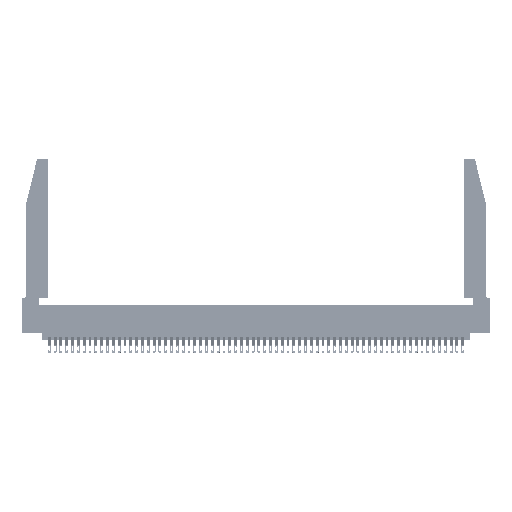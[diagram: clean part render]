
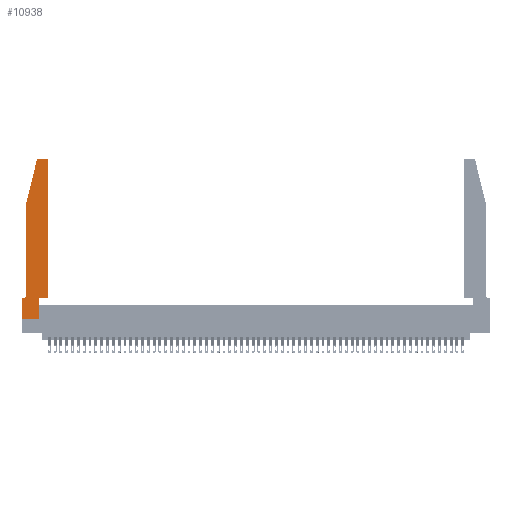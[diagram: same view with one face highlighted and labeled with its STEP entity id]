
A CAD part, top view. The second image highlights one B-rep face of the part: STEP entity #10938.
In plain terms, the highlighted planar face has unit normal (0, 0, 1).
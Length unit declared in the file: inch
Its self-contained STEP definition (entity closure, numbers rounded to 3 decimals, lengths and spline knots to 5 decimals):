
#44 = EDGE_CURVE ( 'NONE', #14950, #2141, #17906, .T. ) ;
#338 = EDGE_CURVE ( 'NONE', #9781, #14950, #34547, .T. ) ;
#500 = ORIENTED_EDGE ( 'NONE', *, *, #44272, .T. ) ;
#587 = DIRECTION ( 'NONE',  ( 1., 0., 0. ) ) ;
#1135 = CARTESIAN_POINT ( 'NONE',  ( 0.0055, 0.35, 0.37 ) ) ;
#1324 = ORIENTED_EDGE ( 'NONE', *, *, #37859, .T. ) ;
#2141 = VERTEX_POINT ( 'NONE', #27934 ) ;
#2411 = EDGE_CURVE ( 'NONE', #54295, #3320, #35051, .T. ) ;
#2538 = ORIENTED_EDGE ( 'NONE', *, *, #2411, .T. ) ;
#2945 = VERTEX_POINT ( 'NONE', #25527 ) ;
#3294 = DIRECTION ( 'NONE',  ( 0., 1., 0. ) ) ;
#3320 = VERTEX_POINT ( 'NONE', #22599 ) ;
#3808 = ORIENTED_EDGE ( 'NONE', *, *, #50352, .T. ) ;
#4042 = CIRCLE ( 'NONE', #40705, 0.03 ) ;
#4461 = VECTOR ( 'NONE', #3294, 39.37008 ) ;
#5425 = CARTESIAN_POINT ( 'NONE',  ( 0., 0.35, 0.37 ) ) ;
#9781 = VERTEX_POINT ( 'NONE', #45982 ) ;
#9807 = EDGE_CURVE ( 'NONE', #54959, #39110, #18823, .T. ) ;
#10004 = CIRCLE ( 'NONE', #13353, 0.07 ) ;
#10031 = CARTESIAN_POINT ( 'NONE',  ( 0.0755, 2., 0.37 ) ) ;
#10104 = CARTESIAN_POINT ( 'NONE',  ( 0.4505, 0.35, 0.37 ) ) ;
#10716 = CARTESIAN_POINT ( 'NONE',  ( 0.25487, 2.72718, 0.37 ) ) ;
#10938 = ADVANCED_FACE ( 'NONE', ( #11097 ), #18618, .T. ) ;
#11097 = FACE_OUTER_BOUND ( 'NONE', #32152, .T. ) ;
#13084 = LINE ( 'NONE', #56034, #25462 ) ;
#13353 = AXIS2_PLACEMENT_3D ( 'NONE', #24108, #41771, #50755 ) ;
#13723 = DIRECTION ( 'NONE',  ( 0., -1., 0. ) ) ;
#14192 = CARTESIAN_POINT ( 'NONE',  ( 0.4505, 0.35, 0.37 ) ) ;
#14578 = VECTOR ( 'NONE', #18341, 39.37008 ) ;
#14950 = VERTEX_POINT ( 'NONE', #10716 ) ;
#15101 = DIRECTION ( 'NONE',  ( 1., 0., 0. ) ) ;
#15201 = LINE ( 'NONE', #34002, #32562 ) ;
#17906 = LINE ( 'NONE', #43061, #54844 ) ;
#17944 = ORIENTED_EDGE ( 'NONE', *, *, #9807, .T. ) ;
#18142 = CARTESIAN_POINT ( 'NONE',  ( 0.284, 2.72, 0.37 ) ) ;
#18341 = DIRECTION ( 'NONE',  ( 0., 1., 0. ) ) ;
#18618 = PLANE ( 'NONE',  #49886 ) ;
#18672 = ORIENTED_EDGE ( 'NONE', *, *, #38114, .T. ) ;
#18814 = DIRECTION ( 'NONE',  ( 0., 0., 1. ) ) ;
#18823 = LINE ( 'NONE', #24023, #29229 ) ;
#18865 = DIRECTION ( 'NONE',  ( 1., 0., 0. ) ) ;
#19531 = DIRECTION ( 'NONE',  ( 0., -1., 0. ) ) ;
#20023 = DIRECTION ( 'NONE',  ( -1., 0., 0. ) ) ;
#20073 = VERTEX_POINT ( 'NONE', #49762 ) ;
#20419 = LINE ( 'NONE', #14192, #51088 ) ;
#21362 = VERTEX_POINT ( 'NONE', #42025 ) ;
#22110 = CARTESIAN_POINT ( 'NONE',  ( 0.2865, 0., 0.37 ) ) ;
#22599 = CARTESIAN_POINT ( 'NONE',  ( 0.4505, 2.72, 0.37 ) ) ;
#23251 = CARTESIAN_POINT ( 'NONE',  ( 0., 0.35, 0.37 ) ) ;
#23853 = CARTESIAN_POINT ( 'NONE',  ( 0., 0., 0.37 ) ) ;
#24023 = CARTESIAN_POINT ( 'NONE',  ( 0., 0., 0.37 ) ) ;
#24108 = CARTESIAN_POINT ( 'NONE',  ( 0.0055, 0.42, 0.37 ) ) ;
#25462 = VECTOR ( 'NONE', #20023, 39.37008 ) ;
#25527 = CARTESIAN_POINT ( 'NONE',  ( 0.2865, 0.35, 0.37 ) ) ;
#25885 = EDGE_CURVE ( 'NONE', #46141, #2945, #50083, .T. ) ;
#26100 = ORIENTED_EDGE ( 'NONE', *, *, #44, .T. ) ;
#27676 = CARTESIAN_POINT ( 'NONE',  ( 0.2865, 0.35, 0.37 ) ) ;
#27758 = DIRECTION ( 'NONE',  ( 1., 0., 0. ) ) ;
#27934 = CARTESIAN_POINT ( 'NONE',  ( 0.0755, 2., 0.37 ) ) ;
#27991 = VECTOR ( 'NONE', #15101, 39.37008 ) ;
#29229 = VECTOR ( 'NONE', #19531, 39.37008 ) ;
#30416 = CARTESIAN_POINT ( 'NONE',  ( 0.4505, 0.35, 0.37 ) ) ;
#31051 = EDGE_CURVE ( 'NONE', #39110, #46141, #41236, .T. ) ;
#31199 = VECTOR ( 'NONE', #13723, 39.37008 ) ;
#31315 = CARTESIAN_POINT ( 'NONE',  ( 0., 0., 0.37 ) ) ;
#31906 = ORIENTED_EDGE ( 'NONE', *, *, #25885, .T. ) ;
#32152 = EDGE_LOOP ( 'NONE', ( #500, #34786, #26100, #49305, #18672, #3808, #17944, #53571, #31906, #1324, #2538, #52257 ) ) ;
#32562 = VECTOR ( 'NONE', #43526, 39.37008 ) ;
#34002 = CARTESIAN_POINT ( 'NONE',  ( 0.2605, 2.75, 0.37 ) ) ;
#34547 = CIRCLE ( 'NONE', #54072, 0.03 ) ;
#34703 = DIRECTION ( 'NONE',  ( -0.239, -0.971, 0. ) ) ;
#34786 = ORIENTED_EDGE ( 'NONE', *, *, #338, .T. ) ;
#35051 = LINE ( 'NONE', #30416, #4461 ) ;
#36725 = CARTESIAN_POINT ( 'NONE',  ( 0.4205, 2.72, 0.37 ) ) ;
#37859 = EDGE_CURVE ( 'NONE', #2945, #54295, #20419, .T. ) ;
#38114 = EDGE_CURVE ( 'NONE', #20073, #42718, #10004, .T. ) ;
#39110 = VERTEX_POINT ( 'NONE', #31315 ) ;
#40524 = EDGE_CURVE ( 'NONE', #2141, #20073, #48653, .T. ) ;
#40705 = AXIS2_PLACEMENT_3D ( 'NONE', #36725, #54868, #18865 ) ;
#41236 = LINE ( 'NONE', #23853, #27991 ) ;
#41771 = DIRECTION ( 'NONE',  ( 0., 0., -1. ) ) ;
#42025 = CARTESIAN_POINT ( 'NONE',  ( 0.4205, 2.75, 0.37 ) ) ;
#42067 = EDGE_CURVE ( 'NONE', #3320, #21362, #4042, .T. ) ;
#42718 = VERTEX_POINT ( 'NONE', #1135 ) ;
#43061 = CARTESIAN_POINT ( 'NONE',  ( 0.0755, 2., 0.37 ) ) ;
#43526 = DIRECTION ( 'NONE',  ( -1., 0., 0. ) ) ;
#44272 = EDGE_CURVE ( 'NONE', #21362, #9781, #15201, .T. ) ;
#45177 = DIRECTION ( 'NONE',  ( 0., 0., 1. ) ) ;
#45982 = CARTESIAN_POINT ( 'NONE',  ( 0.284, 2.75, 0.37 ) ) ;
#46141 = VERTEX_POINT ( 'NONE', #22110 ) ;
#48653 = LINE ( 'NONE', #10031, #31199 ) ;
#49305 = ORIENTED_EDGE ( 'NONE', *, *, #40524, .T. ) ;
#49762 = CARTESIAN_POINT ( 'NONE',  ( 0.0755, 0.42, 0.37 ) ) ;
#49886 = AXIS2_PLACEMENT_3D ( 'NONE', #5425, #18814, #27758 ) ;
#49893 = DIRECTION ( 'NONE',  ( 1., 0., 0. ) ) ;
#50083 = LINE ( 'NONE', #27676, #14578 ) ;
#50352 = EDGE_CURVE ( 'NONE', #42718, #54959, #13084, .T. ) ;
#50755 = DIRECTION ( 'NONE',  ( -1., 0., 0. ) ) ;
#51088 = VECTOR ( 'NONE', #587, 39.37008 ) ;
#52257 = ORIENTED_EDGE ( 'NONE', *, *, #42067, .T. ) ;
#53571 = ORIENTED_EDGE ( 'NONE', *, *, #31051, .T. ) ;
#54072 = AXIS2_PLACEMENT_3D ( 'NONE', #18142, #45177, #49893 ) ;
#54295 = VERTEX_POINT ( 'NONE', #10104 ) ;
#54844 = VECTOR ( 'NONE', #34703, 39.37008 ) ;
#54868 = DIRECTION ( 'NONE',  ( 0., 0., 1. ) ) ;
#54959 = VERTEX_POINT ( 'NONE', #23251 ) ;
#56034 = CARTESIAN_POINT ( 'NONE',  ( 0.0755, 0.35, 0.37 ) ) ;
